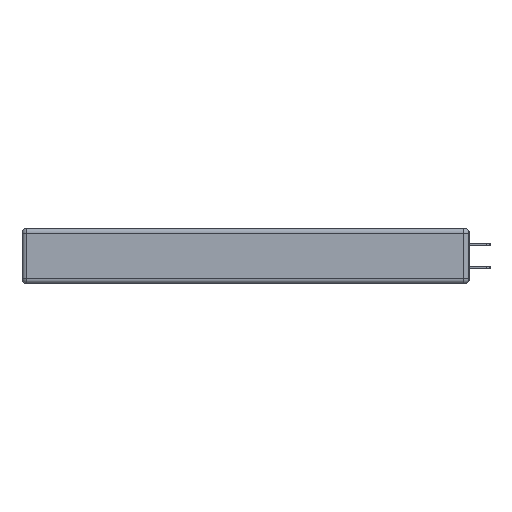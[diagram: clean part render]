
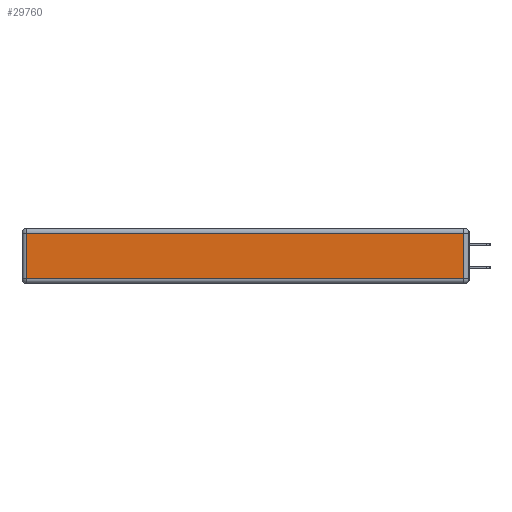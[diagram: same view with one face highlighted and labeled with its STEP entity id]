
A CAD part, left-side view. The second image highlights one B-rep face of the part: STEP entity #29760.
In plain terms, the highlighted planar face has unit normal (-1, 0, 0).
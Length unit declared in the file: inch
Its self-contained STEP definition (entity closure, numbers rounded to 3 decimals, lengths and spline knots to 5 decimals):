
#483 = PLANE ( 'NONE',  #17481 ) ;
#877 = DIRECTION ( 'NONE',  ( 0., -1., 0. ) ) ;
#1087 = VECTOR ( 'NONE', #17975, 39.37008 ) ;
#1837 = VERTEX_POINT ( 'NONE', #11785 ) ;
#2394 = EDGE_CURVE ( 'NONE', #8466, #19632, #22059, .T. ) ;
#3012 = DIRECTION ( 'NONE',  ( 0., 1., 0. ) ) ;
#4931 = DIRECTION ( 'NONE',  ( -1., 0., 0. ) ) ;
#6495 = ORIENTED_EDGE ( 'NONE', *, *, #16063, .T. ) ;
#8380 = CARTESIAN_POINT ( 'NONE',  ( 0., 2.72, -0.343 ) ) ;
#8466 = VERTEX_POINT ( 'NONE', #16137 ) ;
#9652 = CARTESIAN_POINT ( 'NONE',  ( 0., 2.75, -0.03 ) ) ;
#10084 = LINE ( 'NONE', #29295, #26849 ) ;
#11028 = DIRECTION ( 'NONE',  ( 0., 0., 1. ) ) ;
#11785 = CARTESIAN_POINT ( 'NONE',  ( 0., 2.72, -0.03 ) ) ;
#12226 = ORIENTED_EDGE ( 'NONE', *, *, #29912, .T. ) ;
#12405 = VECTOR ( 'NONE', #11028, 39.37008 ) ;
#13084 = ORIENTED_EDGE ( 'NONE', *, *, #15745, .T. ) ;
#13544 = CARTESIAN_POINT ( 'NONE',  ( 0., 0.03, -0.343 ) ) ;
#14533 = DIRECTION ( 'NONE',  ( 0., 0., 1. ) ) ;
#15745 = EDGE_CURVE ( 'NONE', #19632, #1837, #18987, .T. ) ;
#16063 = EDGE_CURVE ( 'NONE', #1837, #16210, #17103, .T. ) ;
#16137 = CARTESIAN_POINT ( 'NONE',  ( 0., 0.03, -0.313 ) ) ;
#16210 = VERTEX_POINT ( 'NONE', #22948 ) ;
#16266 = CARTESIAN_POINT ( 'NONE',  ( 0., 0.03, -0.03 ) ) ;
#17103 = LINE ( 'NONE', #8380, #1087 ) ;
#17481 = AXIS2_PLACEMENT_3D ( 'NONE', #26305, #4931, #14533 ) ;
#17975 = DIRECTION ( 'NONE',  ( 0., 0., -1. ) ) ;
#18987 = LINE ( 'NONE', #9652, #26461 ) ;
#19632 = VERTEX_POINT ( 'NONE', #16266 ) ;
#22059 = LINE ( 'NONE', #13544, #12405 ) ;
#22948 = CARTESIAN_POINT ( 'NONE',  ( 0., 2.72, -0.313 ) ) ;
#23147 = FACE_OUTER_BOUND ( 'NONE', #26611, .T. ) ;
#26305 = CARTESIAN_POINT ( 'NONE',  ( 0., 0., -0.343 ) ) ;
#26461 = VECTOR ( 'NONE', #3012, 39.37008 ) ;
#26611 = EDGE_LOOP ( 'NONE', ( #12226, #29733, #13084, #6495 ) ) ;
#26849 = VECTOR ( 'NONE', #877, 39.37008 ) ;
#29295 = CARTESIAN_POINT ( 'NONE',  ( 0., 0., -0.313 ) ) ;
#29733 = ORIENTED_EDGE ( 'NONE', *, *, #2394, .T. ) ;
#29760 = ADVANCED_FACE ( 'NONE', ( #23147 ), #483, .T. ) ;
#29912 = EDGE_CURVE ( 'NONE', #16210, #8466, #10084, .T. ) ;
